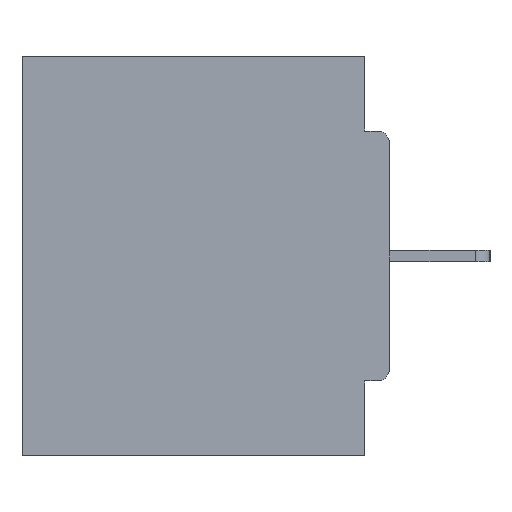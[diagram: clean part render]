
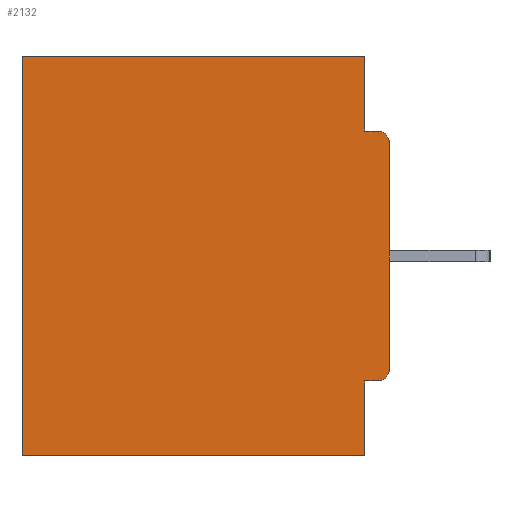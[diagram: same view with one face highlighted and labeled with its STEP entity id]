
A CAD part, left-side view. The second image highlights one B-rep face of the part: STEP entity #2132.
In plain terms, the highlighted planar face has unit normal (-1, 0, 0).
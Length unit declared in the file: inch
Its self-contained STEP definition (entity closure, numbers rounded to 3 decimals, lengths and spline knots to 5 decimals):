
#143 = ORIENTED_EDGE ( 'NONE', *, *, #16788, .T. ) ;
#674 = EDGE_LOOP ( 'NONE', ( #5410, #8486, #21168, #22456, #143, #4842, #9389, #23166, #26515, #10237 ) ) ;
#1230 = CIRCLE ( 'NONE', #21661, 0.015 ) ;
#1379 = FACE_OUTER_BOUND ( 'NONE', #674, .T. ) ;
#2132 = ADVANCED_FACE ( 'NONE', ( #1379 ), #18445, .F. ) ;
#2165 = CARTESIAN_POINT ( 'NONE',  ( 0.298, 0.015, -0.1085 ) ) ;
#2484 = CIRCLE ( 'NONE', #25125, 0.015 ) ;
#3038 = VERTEX_POINT ( 'NONE', #3977 ) ;
#3485 = DIRECTION ( 'NONE',  ( 0., 1., 0. ) ) ;
#3690 = VERTEX_POINT ( 'NONE', #29696 ) ;
#3780 = CARTESIAN_POINT ( 'NONE',  ( 0.298, 0., -0.4065 ) ) ;
#3977 = CARTESIAN_POINT ( 'NONE',  ( 0.298, 0.031, -0.0935 ) ) ;
#4842 = ORIENTED_EDGE ( 'NONE', *, *, #11964, .F. ) ;
#4876 = CARTESIAN_POINT ( 'NONE',  ( 0.298, 0.031, -0.5 ) ) ;
#5034 = VERTEX_POINT ( 'NONE', #26927 ) ;
#5410 = ORIENTED_EDGE ( 'NONE', *, *, #7710, .T. ) ;
#6146 = DIRECTION ( 'NONE',  ( 0., 1., 0. ) ) ;
#6495 = CARTESIAN_POINT ( 'NONE',  ( 0.298, 0.031, -0.5 ) ) ;
#6858 = VERTEX_POINT ( 'NONE', #4876 ) ;
#7086 = VECTOR ( 'NONE', #6146, 39.37008 ) ;
#7272 = EDGE_CURVE ( 'NONE', #5034, #24426, #14430, .T. ) ;
#7573 = CARTESIAN_POINT ( 'NONE',  ( 0.298, 0.015, -0.4065 ) ) ;
#7686 = EDGE_CURVE ( 'NONE', #15216, #6858, #21159, .T. ) ;
#7710 = EDGE_CURVE ( 'NONE', #5034, #3690, #2484, .T. ) ;
#7790 = DIRECTION ( 'NONE',  ( -1., 0., 0. ) ) ;
#7814 = CARTESIAN_POINT ( 'NONE',  ( 0.298, 0., 0. ) ) ;
#8058 = DIRECTION ( 'NONE',  ( 0., 0., -1. ) ) ;
#8174 = AXIS2_PLACEMENT_3D ( 'NONE', #24062, #26788, #27111 ) ;
#8486 = ORIENTED_EDGE ( 'NONE', *, *, #20362, .F. ) ;
#8813 = VECTOR ( 'NONE', #16562, 39.37008 ) ;
#9389 = ORIENTED_EDGE ( 'NONE', *, *, #7686, .F. ) ;
#9859 = CARTESIAN_POINT ( 'NONE',  ( 0.298, 0.46, -0.5 ) ) ;
#10195 = VECTOR ( 'NONE', #22726, 39.37008 ) ;
#10237 = ORIENTED_EDGE ( 'NONE', *, *, #7272, .F. ) ;
#10518 = CARTESIAN_POINT ( 'NONE',  ( 0.298, 0., 0. ) ) ;
#10524 = VERTEX_POINT ( 'NONE', #9859 ) ;
#11060 = DIRECTION ( 'NONE',  ( 0., -1., 0. ) ) ;
#11964 = EDGE_CURVE ( 'NONE', #6858, #10524, #23970, .T. ) ;
#13086 = LINE ( 'NONE', #27068, #17721 ) ;
#13127 = DIRECTION ( 'NONE',  ( 0., 1., 0. ) ) ;
#13362 = DIRECTION ( 'NONE',  ( 0., 0., -1. ) ) ;
#14430 = LINE ( 'NONE', #7814, #25773 ) ;
#15077 = VECTOR ( 'NONE', #13362, 39.37008 ) ;
#15216 = VERTEX_POINT ( 'NONE', #21231 ) ;
#16438 = LINE ( 'NONE', #6495, #10195 ) ;
#16510 = CARTESIAN_POINT ( 'NONE',  ( 0.298, 0.031, 0. ) ) ;
#16562 = DIRECTION ( 'NONE',  ( 0., 0., -1. ) ) ;
#16788 = EDGE_CURVE ( 'NONE', #28437, #10524, #21843, .T. ) ;
#17721 = VECTOR ( 'NONE', #11060, 39.37008 ) ;
#18445 = PLANE ( 'NONE',  #8174 ) ;
#18471 = CARTESIAN_POINT ( 'NONE',  ( 0.298, 0.46, 0. ) ) ;
#18648 = EDGE_CURVE ( 'NONE', #25676, #3038, #16438, .T. ) ;
#20019 = CARTESIAN_POINT ( 'NONE',  ( 0.298, 0., -0.5 ) ) ;
#20243 = CARTESIAN_POINT ( 'NONE',  ( 0.298, 0.46, 0. ) ) ;
#20362 = EDGE_CURVE ( 'NONE', #3038, #3690, #13086, .T. ) ;
#21159 = LINE ( 'NONE', #23457, #8813 ) ;
#21168 = ORIENTED_EDGE ( 'NONE', *, *, #18648, .F. ) ;
#21231 = CARTESIAN_POINT ( 'NONE',  ( 0.298, 0.031, -0.4065 ) ) ;
#21363 = DIRECTION ( 'NONE',  ( -1., 0., 0. ) ) ;
#21661 = AXIS2_PLACEMENT_3D ( 'NONE', #21723, #7790, #23992 ) ;
#21723 = CARTESIAN_POINT ( 'NONE',  ( 0.298, 0.015, -0.3915 ) ) ;
#21843 = LINE ( 'NONE', #20243, #15077 ) ;
#21885 = VECTOR ( 'NONE', #3485, 39.37008 ) ;
#22300 = EDGE_CURVE ( 'NONE', #25676, #28437, #27865, .T. ) ;
#22456 = ORIENTED_EDGE ( 'NONE', *, *, #22300, .T. ) ;
#22542 = VECTOR ( 'NONE', #13127, 39.37008 ) ;
#22726 = DIRECTION ( 'NONE',  ( 0., 0., -1. ) ) ;
#22781 = VERTEX_POINT ( 'NONE', #7573 ) ;
#23166 = ORIENTED_EDGE ( 'NONE', *, *, #29391, .F. ) ;
#23457 = CARTESIAN_POINT ( 'NONE',  ( 0.298, 0.031, -0.5 ) ) ;
#23970 = LINE ( 'NONE', #20019, #22542 ) ;
#23992 = DIRECTION ( 'NONE',  ( 0., 0., -1. ) ) ;
#24062 = CARTESIAN_POINT ( 'NONE',  ( 0.298, 0., 0. ) ) ;
#24426 = VERTEX_POINT ( 'NONE', #27051 ) ;
#24788 = EDGE_CURVE ( 'NONE', #22781, #24426, #1230, .T. ) ;
#25125 = AXIS2_PLACEMENT_3D ( 'NONE', #2165, #21363, #26400 ) ;
#25676 = VERTEX_POINT ( 'NONE', #16510 ) ;
#25773 = VECTOR ( 'NONE', #8058, 39.37008 ) ;
#26221 = LINE ( 'NONE', #3780, #7086 ) ;
#26400 = DIRECTION ( 'NONE',  ( 0., 0., -1. ) ) ;
#26515 = ORIENTED_EDGE ( 'NONE', *, *, #24788, .T. ) ;
#26788 = DIRECTION ( 'NONE',  ( 1., 0., 0. ) ) ;
#26927 = CARTESIAN_POINT ( 'NONE',  ( 0.298, 0., -0.1085 ) ) ;
#27051 = CARTESIAN_POINT ( 'NONE',  ( 0.298, 0., -0.3915 ) ) ;
#27068 = CARTESIAN_POINT ( 'NONE',  ( 0.298, 0., -0.0935 ) ) ;
#27111 = DIRECTION ( 'NONE',  ( 0., 0., -1. ) ) ;
#27865 = LINE ( 'NONE', #10518, #21885 ) ;
#28437 = VERTEX_POINT ( 'NONE', #18471 ) ;
#29391 = EDGE_CURVE ( 'NONE', #22781, #15216, #26221, .T. ) ;
#29696 = CARTESIAN_POINT ( 'NONE',  ( 0.298, 0.015, -0.0935 ) ) ;
